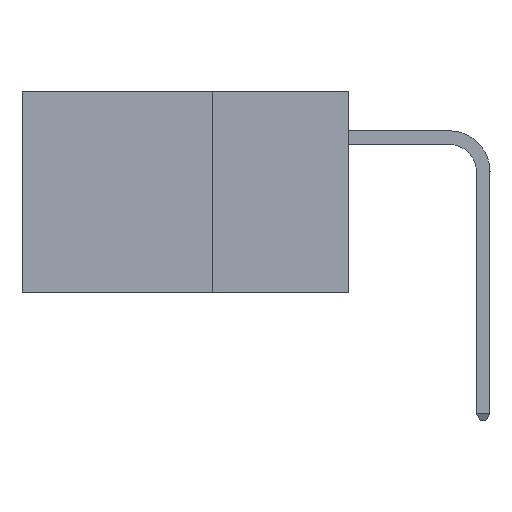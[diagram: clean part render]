
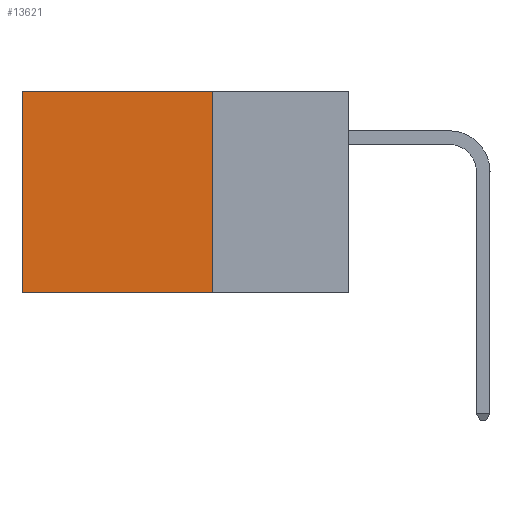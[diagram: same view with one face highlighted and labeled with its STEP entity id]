
A CAD part, left-side view. The second image highlights one B-rep face of the part: STEP entity #13621.
In plain terms, the highlighted planar face has unit normal (-1, 0, 0).
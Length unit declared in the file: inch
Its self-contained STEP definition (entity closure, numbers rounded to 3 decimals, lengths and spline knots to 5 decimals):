
#983 = DIRECTION ( 'NONE',  ( 0., 0., -1. ) ) ;
#2186 = VERTEX_POINT ( 'NONE', #17225 ) ;
#3711 = CARTESIAN_POINT ( 'NONE',  ( 0.2875, 0.25, -0.37 ) ) ;
#5839 = DIRECTION ( 'NONE',  ( 0., 1., 0. ) ) ;
#6662 = LINE ( 'NONE', #19343, #8671 ) ;
#6981 = LINE ( 'NONE', #38515, #22580 ) ;
#8671 = VECTOR ( 'NONE', #31610, 39.37008 ) ;
#9806 = CARTESIAN_POINT ( 'NONE',  ( 0.2875, 0.25, -0.37 ) ) ;
#11097 = VERTEX_POINT ( 'NONE', #9806 ) ;
#11835 = VERTEX_POINT ( 'NONE', #16465 ) ;
#12455 = EDGE_CURVE ( 'NONE', #11097, #11835, #16892, .T. ) ;
#12952 = ORIENTED_EDGE ( 'NONE', *, *, #29910, .T. ) ;
#13621 = ADVANCED_FACE ( 'NONE', ( #28360 ), #35051, .F. ) ;
#15219 = AXIS2_PLACEMENT_3D ( 'NONE', #38088, #19845, #983 ) ;
#16465 = CARTESIAN_POINT ( 'NONE',  ( 0.2875, 0.6, -0.37 ) ) ;
#16892 = LINE ( 'NONE', #3711, #38900 ) ;
#17174 = DIRECTION ( 'NONE',  ( 0., 0., -1. ) ) ;
#17225 = CARTESIAN_POINT ( 'NONE',  ( 0.2875, 0.6, 0. ) ) ;
#18743 = EDGE_CURVE ( 'NONE', #2186, #11835, #6662, .T. ) ;
#19343 = CARTESIAN_POINT ( 'NONE',  ( 0.2875, 0.6, 0. ) ) ;
#19845 = DIRECTION ( 'NONE',  ( 1., 0., 0. ) ) ;
#21430 = CARTESIAN_POINT ( 'NONE',  ( 0.2875, 0.25, 0. ) ) ;
#22580 = VECTOR ( 'NONE', #17174, 39.37008 ) ;
#22761 = CARTESIAN_POINT ( 'NONE',  ( 0.2875, 0.25, 0. ) ) ;
#23401 = ORIENTED_EDGE ( 'NONE', *, *, #18743, .T. ) ;
#26804 = EDGE_LOOP ( 'NONE', ( #23401, #31965, #31514, #12952 ) ) ;
#28360 = FACE_OUTER_BOUND ( 'NONE', #26804, .T. ) ;
#29910 = EDGE_CURVE ( 'NONE', #31014, #2186, #39281, .T. ) ;
#30930 = EDGE_CURVE ( 'NONE', #31014, #11097, #6981, .T. ) ;
#31014 = VERTEX_POINT ( 'NONE', #22761 ) ;
#31220 = VECTOR ( 'NONE', #5839, 39.37008 ) ;
#31514 = ORIENTED_EDGE ( 'NONE', *, *, #30930, .F. ) ;
#31535 = DIRECTION ( 'NONE',  ( 0., 1., 0. ) ) ;
#31610 = DIRECTION ( 'NONE',  ( 0., 0., -1. ) ) ;
#31965 = ORIENTED_EDGE ( 'NONE', *, *, #12455, .F. ) ;
#35051 = PLANE ( 'NONE',  #15219 ) ;
#38088 = CARTESIAN_POINT ( 'NONE',  ( 0.2875, 0.25, 0. ) ) ;
#38515 = CARTESIAN_POINT ( 'NONE',  ( 0.2875, 0.25, 0. ) ) ;
#38900 = VECTOR ( 'NONE', #31535, 39.37008 ) ;
#39281 = LINE ( 'NONE', #21430, #31220 ) ;
